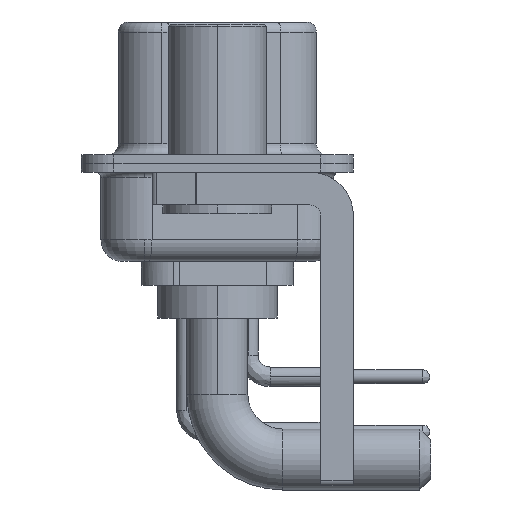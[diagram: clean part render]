
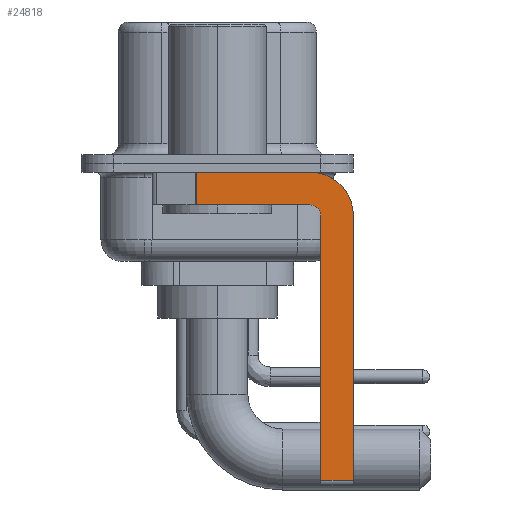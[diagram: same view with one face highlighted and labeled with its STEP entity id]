
A CAD part, left-side view. The second image highlights one B-rep face of the part: STEP entity #24818.
In plain terms, the highlighted planar face has unit normal (-1, 0, 0).
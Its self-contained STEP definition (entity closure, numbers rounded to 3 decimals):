
#594 = PLANE ( 'NONE',  #17208 ) ;
#662 = ORIENTED_EDGE ( 'NONE', *, *, #7503, .F. ) ;
#730 = CIRCLE ( 'NONE', #11725, 0.5 ) ;
#1562 = EDGE_LOOP ( 'NONE', ( #4123, #22463, #14368, #22123, #9522, #25227, #19799, #662 ) ) ;
#2098 = CARTESIAN_POINT ( 'NONE',  ( -2.9, -6.25, -14.55 ) ) ;
#2522 = VERTEX_POINT ( 'NONE', #8582 ) ;
#3312 = EDGE_CURVE ( 'NONE', #7841, #5687, #11714, .T. ) ;
#3490 = LINE ( 'NONE', #19750, #5319 ) ;
#4123 = ORIENTED_EDGE ( 'NONE', *, *, #8859, .F. ) ;
#4252 = VERTEX_POINT ( 'NONE', #19905 ) ;
#5319 = VECTOR ( 'NONE', #9731, 1000. ) ;
#5463 = VERTEX_POINT ( 'NONE', #6896 ) ;
#5476 = VECTOR ( 'NONE', #15462, 1000. ) ;
#5622 = VERTEX_POINT ( 'NONE', #19947 ) ;
#5687 = VERTEX_POINT ( 'NONE', #2098 ) ;
#6896 = CARTESIAN_POINT ( 'NONE',  ( -2.9, -6.25, -2.4 ) ) ;
#7503 = EDGE_CURVE ( 'NONE', #5622, #5463, #17810, .T. ) ;
#7680 = LINE ( 'NONE', #19309, #22523 ) ;
#7841 = VERTEX_POINT ( 'NONE', #19364 ) ;
#8297 = CARTESIAN_POINT ( 'NONE',  ( -2.9, -6.25, -2.4 ) ) ;
#8405 = DIRECTION ( 'NONE',  ( 0., 0., -1. ) ) ;
#8500 = LINE ( 'NONE', #21038, #19168 ) ;
#8582 = CARTESIAN_POINT ( 'NONE',  ( -2.9, -4.25, -1.9 ) ) ;
#8713 = EDGE_CURVE ( 'NONE', #7841, #25364, #8500, .T. ) ;
#8859 = EDGE_CURVE ( 'NONE', #14444, #5622, #7680, .T. ) ;
#9522 = ORIENTED_EDGE ( 'NONE', *, *, #8713, .F. ) ;
#9731 = DIRECTION ( 'NONE',  ( 0., 0., -1. ) ) ;
#10027 = VECTOR ( 'NONE', #20427, 1000. ) ;
#10280 = DIRECTION ( 'NONE',  ( 1., 0., 0. ) ) ;
#10628 = EDGE_CURVE ( 'NONE', #14444, #4252, #3490, .T. ) ;
#10644 = FACE_OUTER_BOUND ( 'NONE', #1562, .T. ) ;
#11144 = DIRECTION ( 'NONE',  ( 0., -1., 0. ) ) ;
#11714 = LINE ( 'NONE', #19745, #16884 ) ;
#11725 = AXIS2_PLACEMENT_3D ( 'NONE', #13621, #19798, #17938 ) ;
#12475 = DIRECTION ( 'NONE',  ( 0., 0., 1. ) ) ;
#13621 = CARTESIAN_POINT ( 'NONE',  ( -2.9, -4.25, -2.4 ) ) ;
#13657 = CARTESIAN_POINT ( 'NONE',  ( -2.9, 0.978, -0.4 ) ) ;
#13761 = EDGE_CURVE ( 'NONE', #25364, #2522, #730, .T. ) ;
#14368 = ORIENTED_EDGE ( 'NONE', *, *, #14970, .F. ) ;
#14444 = VERTEX_POINT ( 'NONE', #13657 ) ;
#14970 = EDGE_CURVE ( 'NONE', #2522, #4252, #15082, .T. ) ;
#15082 = LINE ( 'NONE', #21131, #5476 ) ;
#15091 = CARTESIAN_POINT ( 'NONE',  ( -2.9, -4.75, -2.4 ) ) ;
#15462 = DIRECTION ( 'NONE',  ( 0., 1., 0. ) ) ;
#15786 = DIRECTION ( 'NONE',  ( 0., -1., 0. ) ) ;
#16704 = CARTESIAN_POINT ( 'NONE',  ( -2.9, -4.25, -2.4 ) ) ;
#16884 = VECTOR ( 'NONE', #15786, 1000. ) ;
#17208 = AXIS2_PLACEMENT_3D ( 'NONE', #16704, #24482, #8405 ) ;
#17810 = CIRCLE ( 'NONE', #19934, 2. ) ;
#17938 = DIRECTION ( 'NONE',  ( 0., 0., 1. ) ) ;
#18304 = DIRECTION ( 'NONE',  ( 0., 0., -1. ) ) ;
#19168 = VECTOR ( 'NONE', #12475, 1000. ) ;
#19309 = CARTESIAN_POINT ( 'NONE',  ( -2.9, 3., -0.4 ) ) ;
#19364 = CARTESIAN_POINT ( 'NONE',  ( -2.9, -4.75, -14.55 ) ) ;
#19745 = CARTESIAN_POINT ( 'NONE',  ( -2.9, -4.25, -14.55 ) ) ;
#19750 = CARTESIAN_POINT ( 'NONE',  ( -2.9, 0.978, -1.9 ) ) ;
#19798 = DIRECTION ( 'NONE',  ( -1., 0., 0. ) ) ;
#19799 = ORIENTED_EDGE ( 'NONE', *, *, #24351, .F. ) ;
#19905 = CARTESIAN_POINT ( 'NONE',  ( -2.9, 0.978, -1.9 ) ) ;
#19934 = AXIS2_PLACEMENT_3D ( 'NONE', #24248, #10280, #18304 ) ;
#19947 = CARTESIAN_POINT ( 'NONE',  ( -2.9, -4.25, -0.4 ) ) ;
#20427 = DIRECTION ( 'NONE',  ( 0., 0., -1. ) ) ;
#21038 = CARTESIAN_POINT ( 'NONE',  ( -2.9, -4.75, -14.8 ) ) ;
#21131 = CARTESIAN_POINT ( 'NONE',  ( -2.9, -4.25, -1.9 ) ) ;
#22123 = ORIENTED_EDGE ( 'NONE', *, *, #13761, .F. ) ;
#22393 = LINE ( 'NONE', #8297, #10027 ) ;
#22463 = ORIENTED_EDGE ( 'NONE', *, *, #10628, .T. ) ;
#22523 = VECTOR ( 'NONE', #11144, 1000. ) ;
#24248 = CARTESIAN_POINT ( 'NONE',  ( -2.9, -4.25, -2.4 ) ) ;
#24351 = EDGE_CURVE ( 'NONE', #5463, #5687, #22393, .T. ) ;
#24482 = DIRECTION ( 'NONE',  ( 1., 0., 0. ) ) ;
#24818 = ADVANCED_FACE ( 'NONE', ( #10644 ), #594, .F. ) ;
#25227 = ORIENTED_EDGE ( 'NONE', *, *, #3312, .T. ) ;
#25364 = VERTEX_POINT ( 'NONE', #15091 ) ;
